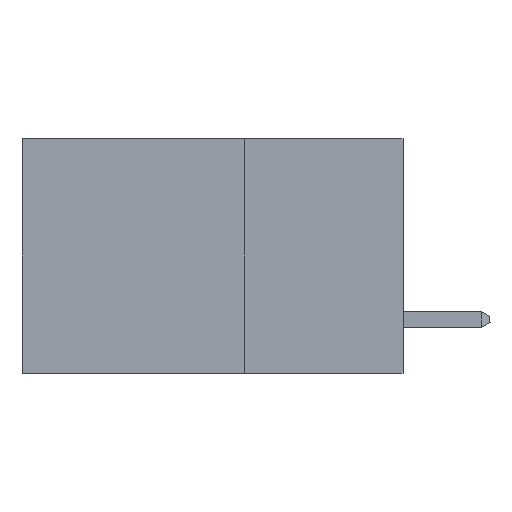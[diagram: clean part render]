
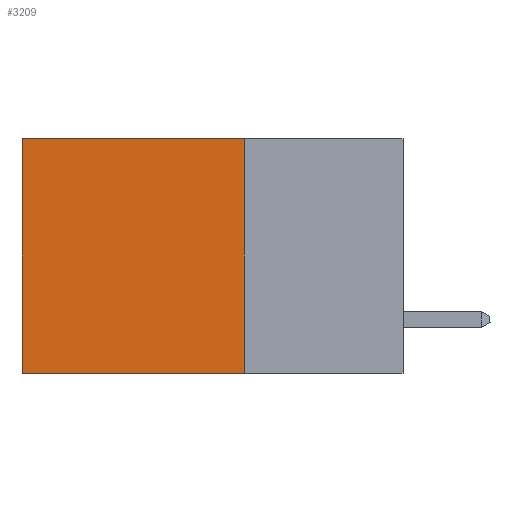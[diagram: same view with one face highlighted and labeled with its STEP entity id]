
A CAD part, left-side view. The second image highlights one B-rep face of the part: STEP entity #3209.
In plain terms, the highlighted planar face has unit normal (-1, 0, 0).
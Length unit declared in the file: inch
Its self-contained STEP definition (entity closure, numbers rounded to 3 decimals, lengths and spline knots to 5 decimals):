
#222 = EDGE_CURVE ( 'NONE', #43983, #12380, #36065, .T. ) ;
#935 = ORIENTED_EDGE ( 'NONE', *, *, #5616, .F. ) ;
#2582 = FACE_OUTER_BOUND ( 'NONE', #4082, .T. ) ;
#2698 = CARTESIAN_POINT ( 'NONE',  ( 0.2875, 0.25, 0. ) ) ;
#3209 = ADVANCED_FACE ( 'NONE', ( #2582 ), #13901, .F. ) ;
#4082 = EDGE_LOOP ( 'NONE', ( #12747, #18575, #935, #40656 ) ) ;
#4641 = VECTOR ( 'NONE', #38344, 39.37008 ) ;
#5616 = EDGE_CURVE ( 'NONE', #43983, #20071, #39928, .T. ) ;
#6648 = CARTESIAN_POINT ( 'NONE',  ( 0.2875, 0.25, -0.37 ) ) ;
#6768 = VECTOR ( 'NONE', #35896, 39.37008 ) ;
#6971 = DIRECTION ( 'NONE',  ( 0., 0., -1. ) ) ;
#8670 = CARTESIAN_POINT ( 'NONE',  ( 0.2875, 0.25, 0. ) ) ;
#11257 = EDGE_CURVE ( 'NONE', #20071, #38732, #16247, .T. ) ;
#12380 = VERTEX_POINT ( 'NONE', #16383 ) ;
#12747 = ORIENTED_EDGE ( 'NONE', *, *, #44442, .T. ) ;
#13339 = CARTESIAN_POINT ( 'NONE',  ( 0.2875, 0.25, -0.37 ) ) ;
#13901 = PLANE ( 'NONE',  #29857 ) ;
#16247 = LINE ( 'NONE', #6648, #4641 ) ;
#16383 = CARTESIAN_POINT ( 'NONE',  ( 0.2875, 0.6, 0. ) ) ;
#18575 = ORIENTED_EDGE ( 'NONE', *, *, #11257, .F. ) ;
#19806 = DIRECTION ( 'NONE',  ( 0., 0., -1. ) ) ;
#20071 = VERTEX_POINT ( 'NONE', #13339 ) ;
#21280 = CARTESIAN_POINT ( 'NONE',  ( 0.2875, 0.6, -0.37 ) ) ;
#21649 = VECTOR ( 'NONE', #19806, 39.37008 ) ;
#24705 = CARTESIAN_POINT ( 'NONE',  ( 0.2875, 0.25, 0. ) ) ;
#29857 = AXIS2_PLACEMENT_3D ( 'NONE', #24705, #35110, #6971 ) ;
#33254 = VECTOR ( 'NONE', #42363, 39.37008 ) ;
#35110 = DIRECTION ( 'NONE',  ( 1., 0., 0. ) ) ;
#35896 = DIRECTION ( 'NONE',  ( 0., 1., 0. ) ) ;
#36065 = LINE ( 'NONE', #2698, #6768 ) ;
#37739 = CARTESIAN_POINT ( 'NONE',  ( 0.2875, 0.25, 0. ) ) ;
#38344 = DIRECTION ( 'NONE',  ( 0., 1., 0. ) ) ;
#38732 = VERTEX_POINT ( 'NONE', #21280 ) ;
#38808 = CARTESIAN_POINT ( 'NONE',  ( 0.2875, 0.6, 0. ) ) ;
#39328 = LINE ( 'NONE', #38808, #33254 ) ;
#39928 = LINE ( 'NONE', #37739, #21649 ) ;
#40656 = ORIENTED_EDGE ( 'NONE', *, *, #222, .T. ) ;
#42363 = DIRECTION ( 'NONE',  ( 0., 0., -1. ) ) ;
#43983 = VERTEX_POINT ( 'NONE', #8670 ) ;
#44442 = EDGE_CURVE ( 'NONE', #12380, #38732, #39328, .T. ) ;
